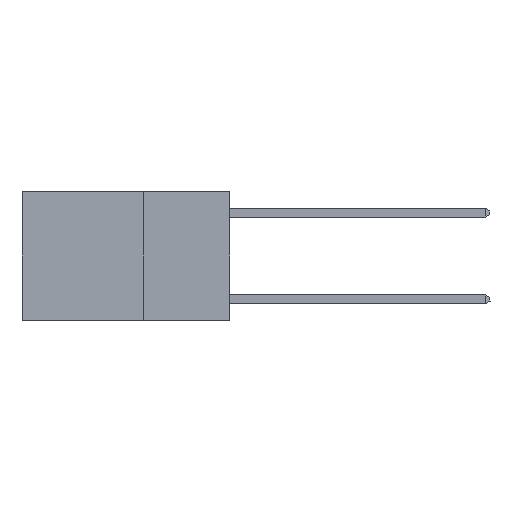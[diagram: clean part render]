
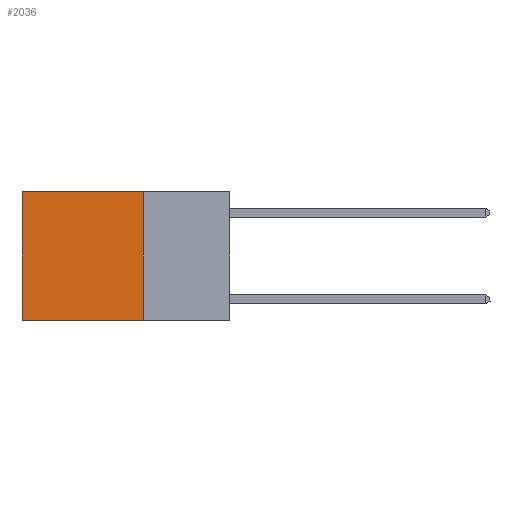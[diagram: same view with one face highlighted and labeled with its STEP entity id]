
A CAD part, left-side view. The second image highlights one B-rep face of the part: STEP entity #2036.
In plain terms, the highlighted planar face has unit normal (-1, 0, 0).
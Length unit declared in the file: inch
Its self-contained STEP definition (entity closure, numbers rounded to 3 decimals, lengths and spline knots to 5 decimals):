
#252 = DIRECTION ( 'NONE',  ( 0., 0., -1. ) ) ;
#740 = EDGE_CURVE ( 'NONE', #4121, #8114, #4364, .T. ) ;
#1235 = ORIENTED_EDGE ( 'NONE', *, *, #8175, .T. ) ;
#1581 = DIRECTION ( 'NONE',  ( 1., 0., 0. ) ) ;
#1787 = CARTESIAN_POINT ( 'NONE',  ( 0.2625, 0.25, 0. ) ) ;
#2036 = ADVANCED_FACE ( 'NONE', ( #11478 ), #4667, .F. ) ;
#2395 = DIRECTION ( 'NONE',  ( 0., 1., 0. ) ) ;
#3131 = EDGE_CURVE ( 'NONE', #4121, #8698, #11806, .T. ) ;
#3924 = AXIS2_PLACEMENT_3D ( 'NONE', #9760, #1581, #8153 ) ;
#3983 = DIRECTION ( 'NONE',  ( 0., 1., 0. ) ) ;
#4121 = VERTEX_POINT ( 'NONE', #10663 ) ;
#4364 = LINE ( 'NONE', #1787, #8677 ) ;
#4572 = CARTESIAN_POINT ( 'NONE',  ( 0.2625, 0.6, 0. ) ) ;
#4667 = PLANE ( 'NONE',  #3924 ) ;
#4705 = ORIENTED_EDGE ( 'NONE', *, *, #5794, .F. ) ;
#5274 = CARTESIAN_POINT ( 'NONE',  ( 0.2625, 0.25, 0. ) ) ;
#5677 = CARTESIAN_POINT ( 'NONE',  ( 0.2625, 0.6, -0.37 ) ) ;
#5794 = EDGE_CURVE ( 'NONE', #8698, #8990, #11386, .T. ) ;
#6191 = EDGE_LOOP ( 'NONE', ( #1235, #4705, #8146, #11887 ) ) ;
#7002 = VECTOR ( 'NONE', #2395, 39.37008 ) ;
#7193 = CARTESIAN_POINT ( 'NONE',  ( 0.2625, 0.25, -0.37 ) ) ;
#7451 = VECTOR ( 'NONE', #9503, 39.37008 ) ;
#8114 = VERTEX_POINT ( 'NONE', #4572 ) ;
#8146 = ORIENTED_EDGE ( 'NONE', *, *, #3131, .F. ) ;
#8153 = DIRECTION ( 'NONE',  ( 0., 0., -1. ) ) ;
#8175 = EDGE_CURVE ( 'NONE', #8114, #8990, #10970, .T. ) ;
#8677 = VECTOR ( 'NONE', #3983, 39.37008 ) ;
#8698 = VERTEX_POINT ( 'NONE', #7193 ) ;
#8818 = VECTOR ( 'NONE', #252, 39.37008 ) ;
#8990 = VERTEX_POINT ( 'NONE', #5677 ) ;
#9503 = DIRECTION ( 'NONE',  ( 0., 0., -1. ) ) ;
#9583 = CARTESIAN_POINT ( 'NONE',  ( 0.2625, 0.25, -0.37 ) ) ;
#9760 = CARTESIAN_POINT ( 'NONE',  ( 0.2625, 0.25, 0. ) ) ;
#10663 = CARTESIAN_POINT ( 'NONE',  ( 0.2625, 0.25, 0. ) ) ;
#10970 = LINE ( 'NONE', #11292, #8818 ) ;
#11292 = CARTESIAN_POINT ( 'NONE',  ( 0.2625, 0.6, 0. ) ) ;
#11386 = LINE ( 'NONE', #9583, #7002 ) ;
#11478 = FACE_OUTER_BOUND ( 'NONE', #6191, .T. ) ;
#11806 = LINE ( 'NONE', #5274, #7451 ) ;
#11887 = ORIENTED_EDGE ( 'NONE', *, *, #740, .T. ) ;
